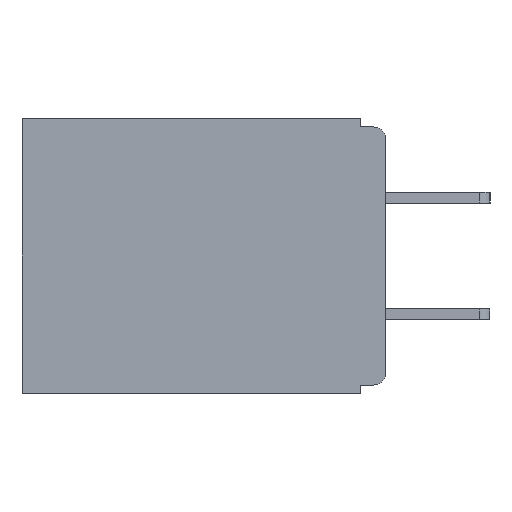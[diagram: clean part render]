
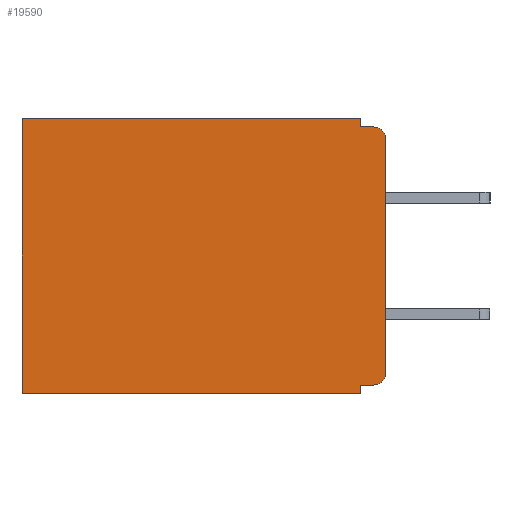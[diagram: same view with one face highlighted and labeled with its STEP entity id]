
A CAD part, left-side view. The second image highlights one B-rep face of the part: STEP entity #19590.
In plain terms, the highlighted planar face has unit normal (-1, 0, 0).
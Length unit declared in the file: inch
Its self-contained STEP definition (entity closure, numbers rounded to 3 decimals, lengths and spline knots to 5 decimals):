
#131 = VECTOR ( 'NONE', #8950, 39.37008 ) ;
#148 = EDGE_CURVE ( 'NONE', #20625, #13698, #22067, .T. ) ;
#170 = ORIENTED_EDGE ( 'NONE', *, *, #3071, .T. ) ;
#355 = DIRECTION ( 'NONE',  ( 1., 0., 0. ) ) ;
#1549 = ORIENTED_EDGE ( 'NONE', *, *, #13418, .F. ) ;
#1959 = CARTESIAN_POINT ( 'NONE',  ( 0.3, 0.031, -0.32 ) ) ;
#2336 = CARTESIAN_POINT ( 'NONE',  ( 0.3, 0.031, 0. ) ) ;
#2836 = VERTEX_POINT ( 'NONE', #1959 ) ;
#3071 = EDGE_CURVE ( 'NONE', #19232, #25454, #13890, .T. ) ;
#3583 = ORIENTED_EDGE ( 'NONE', *, *, #23547, .F. ) ;
#5017 = VECTOR ( 'NONE', #17715, 39.37008 ) ;
#5943 = DIRECTION ( 'NONE',  ( -1., 0., 0. ) ) ;
#6035 = CARTESIAN_POINT ( 'NONE',  ( 0.3, 0.031, -0.01 ) ) ;
#6396 = EDGE_LOOP ( 'NONE', ( #27657, #14610, #23217, #11327, #10863, #10166, #3583, #8132, #1549, #170 ) ) ;
#6785 = EDGE_CURVE ( 'NONE', #20806, #20625, #11255, .T. ) ;
#6938 = LINE ( 'NONE', #22485, #18439 ) ;
#7124 = AXIS2_PLACEMENT_3D ( 'NONE', #13539, #355, #15707 ) ;
#7155 = VERTEX_POINT ( 'NONE', #17347 ) ;
#7562 = EDGE_CURVE ( 'NONE', #7155, #23287, #14998, .T. ) ;
#7598 = VERTEX_POINT ( 'NONE', #6035 ) ;
#7889 = LINE ( 'NONE', #24635, #14398 ) ;
#8132 = ORIENTED_EDGE ( 'NONE', *, *, #10653, .F. ) ;
#8378 = LINE ( 'NONE', #25189, #19159 ) ;
#8950 = DIRECTION ( 'NONE',  ( 0., 0., -1. ) ) ;
#9121 = PLANE ( 'NONE',  #7124 ) ;
#9693 = VECTOR ( 'NONE', #21886, 39.37008 ) ;
#9866 = VECTOR ( 'NONE', #24644, 39.37008 ) ;
#10166 = ORIENTED_EDGE ( 'NONE', *, *, #148, .T. ) ;
#10558 = CARTESIAN_POINT ( 'NONE',  ( 0.3, 0.437, -0.33 ) ) ;
#10653 = EDGE_CURVE ( 'NONE', #2836, #25693, #17531, .T. ) ;
#10863 = ORIENTED_EDGE ( 'NONE', *, *, #6785, .T. ) ;
#11255 = LINE ( 'NONE', #16217, #9866 ) ;
#11327 = ORIENTED_EDGE ( 'NONE', *, *, #12138, .F. ) ;
#11863 = DIRECTION ( 'NONE',  ( 0., 0., -1. ) ) ;
#12138 = EDGE_CURVE ( 'NONE', #20806, #7598, #15516, .T. ) ;
#12566 = CARTESIAN_POINT ( 'NONE',  ( 0.3, 0.437, -0.33 ) ) ;
#13418 = EDGE_CURVE ( 'NONE', #19232, #2836, #6938, .T. ) ;
#13539 = CARTESIAN_POINT ( 'NONE',  ( 0.3, 0., -0.33 ) ) ;
#13698 = VERTEX_POINT ( 'NONE', #10558 ) ;
#13890 = CIRCLE ( 'NONE', #21979, 0.015 ) ;
#14398 = VECTOR ( 'NONE', #11863, 39.37008 ) ;
#14610 = ORIENTED_EDGE ( 'NONE', *, *, #7562, .T. ) ;
#14998 = CIRCLE ( 'NONE', #24004, 0.015 ) ;
#15516 = LINE ( 'NONE', #2336, #9693 ) ;
#15707 = DIRECTION ( 'NONE',  ( 0., 0., -1. ) ) ;
#15892 = CARTESIAN_POINT ( 'NONE',  ( 0.3, 0.015, -0.305 ) ) ;
#16010 = LINE ( 'NONE', #17615, #5017 ) ;
#16217 = CARTESIAN_POINT ( 'NONE',  ( 0.3, 0., 0. ) ) ;
#16784 = DIRECTION ( 'NONE',  ( -1., 0., 0. ) ) ;
#17347 = CARTESIAN_POINT ( 'NONE',  ( 0.3, 0., -0.025 ) ) ;
#17531 = LINE ( 'NONE', #26047, #131 ) ;
#17615 = CARTESIAN_POINT ( 'NONE',  ( 0.3, 0., -0.33 ) ) ;
#17698 = DIRECTION ( 'NONE',  ( 0., 0., -1. ) ) ;
#17715 = DIRECTION ( 'NONE',  ( 0., 1., 0. ) ) ;
#18439 = VECTOR ( 'NONE', #26588, 39.37008 ) ;
#18917 = CARTESIAN_POINT ( 'NONE',  ( 0.3, 0.015, -0.025 ) ) ;
#19159 = VECTOR ( 'NONE', #27277, 39.37008 ) ;
#19232 = VERTEX_POINT ( 'NONE', #24773 ) ;
#19590 = ADVANCED_FACE ( 'NONE', ( #25150 ), #9121, .F. ) ;
#19697 = CARTESIAN_POINT ( 'NONE',  ( 0.3, 0.031, 0. ) ) ;
#20451 = DIRECTION ( 'NONE',  ( 0., 0., -1. ) ) ;
#20565 = EDGE_CURVE ( 'NONE', #7598, #23287, #8378, .T. ) ;
#20625 = VERTEX_POINT ( 'NONE', #23331 ) ;
#20735 = VECTOR ( 'NONE', #20451, 39.37008 ) ;
#20806 = VERTEX_POINT ( 'NONE', #19697 ) ;
#21075 = DIRECTION ( 'NONE',  ( 0., 0., -1. ) ) ;
#21861 = CARTESIAN_POINT ( 'NONE',  ( 0.3, 0., -0.305 ) ) ;
#21886 = DIRECTION ( 'NONE',  ( 0., 0., -1. ) ) ;
#21979 = AXIS2_PLACEMENT_3D ( 'NONE', #15892, #16784, #17698 ) ;
#22067 = LINE ( 'NONE', #12566, #20735 ) ;
#22485 = CARTESIAN_POINT ( 'NONE',  ( 0.3, 0., -0.32 ) ) ;
#22603 = CARTESIAN_POINT ( 'NONE',  ( 0.3, 0.031, -0.33 ) ) ;
#23217 = ORIENTED_EDGE ( 'NONE', *, *, #20565, .F. ) ;
#23287 = VERTEX_POINT ( 'NONE', #27349 ) ;
#23331 = CARTESIAN_POINT ( 'NONE',  ( 0.3, 0.437, 0. ) ) ;
#23547 = EDGE_CURVE ( 'NONE', #25693, #13698, #16010, .T. ) ;
#24004 = AXIS2_PLACEMENT_3D ( 'NONE', #18917, #5943, #21075 ) ;
#24635 = CARTESIAN_POINT ( 'NONE',  ( 0.3, 0., -0.33 ) ) ;
#24644 = DIRECTION ( 'NONE',  ( 0., 1., 0. ) ) ;
#24773 = CARTESIAN_POINT ( 'NONE',  ( 0.3, 0.015, -0.32 ) ) ;
#25150 = FACE_OUTER_BOUND ( 'NONE', #6396, .T. ) ;
#25189 = CARTESIAN_POINT ( 'NONE',  ( 0.3, 0., -0.01 ) ) ;
#25454 = VERTEX_POINT ( 'NONE', #21861 ) ;
#25693 = VERTEX_POINT ( 'NONE', #22603 ) ;
#26047 = CARTESIAN_POINT ( 'NONE',  ( 0.3, 0.031, -0.33 ) ) ;
#26588 = DIRECTION ( 'NONE',  ( 0., 1., 0. ) ) ;
#27277 = DIRECTION ( 'NONE',  ( 0., -1., 0. ) ) ;
#27349 = CARTESIAN_POINT ( 'NONE',  ( 0.3, 0.015, -0.01 ) ) ;
#27600 = EDGE_CURVE ( 'NONE', #7155, #25454, #7889, .T. ) ;
#27657 = ORIENTED_EDGE ( 'NONE', *, *, #27600, .F. ) ;
